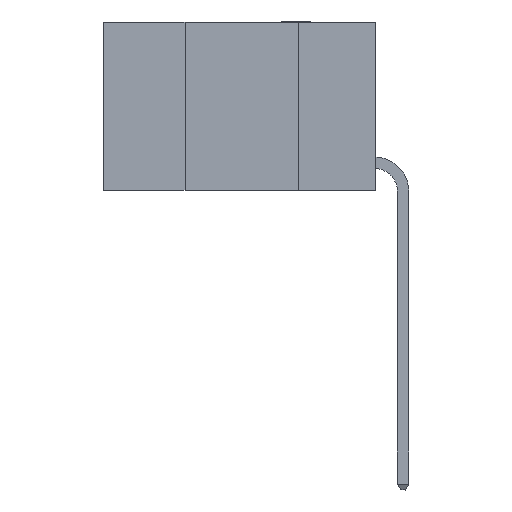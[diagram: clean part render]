
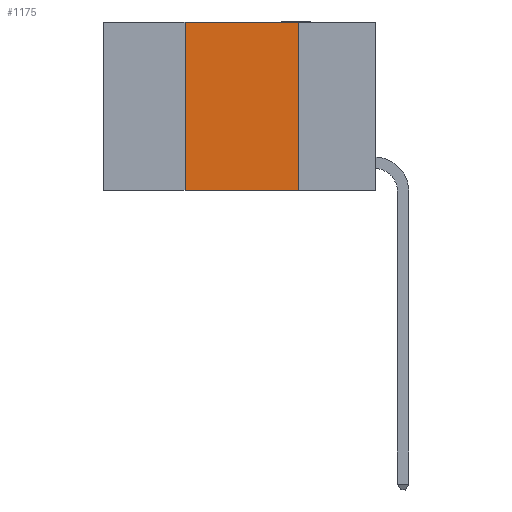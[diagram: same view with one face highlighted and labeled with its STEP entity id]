
A CAD part, left-side view. The second image highlights one B-rep face of the part: STEP entity #1175.
In plain terms, the highlighted planar face has unit normal (-1, 0, 0).
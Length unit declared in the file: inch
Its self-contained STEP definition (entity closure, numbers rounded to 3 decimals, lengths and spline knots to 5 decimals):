
#90 = FACE_OUTER_BOUND ( 'NONE', #10176, .T. ) ;
#216 = VERTEX_POINT ( 'NONE', #8531 ) ;
#694 = CARTESIAN_POINT ( 'NONE',  ( 0., 0.6, 0. ) ) ;
#1175 = ADVANCED_FACE ( 'NONE', ( #90 ), #14462, .F. ) ;
#1737 = VECTOR ( 'NONE', #1869, 39.37008 ) ;
#1763 = LINE ( 'NONE', #4527, #13417 ) ;
#1869 = DIRECTION ( 'NONE',  ( 0., -1., 0. ) ) ;
#3248 = EDGE_CURVE ( 'NONE', #9612, #3502, #7787, .T. ) ;
#3502 = VERTEX_POINT ( 'NONE', #4866 ) ;
#4141 = DIRECTION ( 'NONE',  ( 0., -1., 0. ) ) ;
#4346 = VECTOR ( 'NONE', #9895, 39.37008 ) ;
#4527 = CARTESIAN_POINT ( 'NONE',  ( 0., 0.17, 0. ) ) ;
#4866 = CARTESIAN_POINT ( 'NONE',  ( 0., 0.42, 0. ) ) ;
#6648 = ORIENTED_EDGE ( 'NONE', *, *, #3248, .F. ) ;
#7002 = EDGE_CURVE ( 'NONE', #3502, #216, #7847, .T. ) ;
#7080 = ORIENTED_EDGE ( 'NONE', *, *, #12931, .T. ) ;
#7787 = LINE ( 'NONE', #9945, #4346 ) ;
#7847 = LINE ( 'NONE', #694, #1737 ) ;
#7887 = EDGE_CURVE ( 'NONE', #216, #13329, #1763, .T. ) ;
#8531 = CARTESIAN_POINT ( 'NONE',  ( 0., 0.17, 0. ) ) ;
#8614 = LINE ( 'NONE', #12032, #14479 ) ;
#9342 = DIRECTION ( 'NONE',  ( 0., 0., -1. ) ) ;
#9573 = CARTESIAN_POINT ( 'NONE',  ( 0., 0.42, -0.37 ) ) ;
#9612 = VERTEX_POINT ( 'NONE', #9573 ) ;
#9776 = DIRECTION ( 'NONE',  ( 1., 0., 0. ) ) ;
#9895 = DIRECTION ( 'NONE',  ( 0., 0., 1. ) ) ;
#9945 = CARTESIAN_POINT ( 'NONE',  ( 0., 0.42, 0. ) ) ;
#10176 = EDGE_LOOP ( 'NONE', ( #10765, #11463, #6648, #7080 ) ) ;
#10345 = CARTESIAN_POINT ( 'NONE',  ( 0., 0.6, 0. ) ) ;
#10765 = ORIENTED_EDGE ( 'NONE', *, *, #7887, .F. ) ;
#11463 = ORIENTED_EDGE ( 'NONE', *, *, #7002, .F. ) ;
#11574 = CARTESIAN_POINT ( 'NONE',  ( 0., 0.17, -0.37 ) ) ;
#12032 = CARTESIAN_POINT ( 'NONE',  ( 0., 0.6, -0.37 ) ) ;
#12931 = EDGE_CURVE ( 'NONE', #9612, #13329, #8614, .T. ) ;
#13329 = VERTEX_POINT ( 'NONE', #11574 ) ;
#13417 = VECTOR ( 'NONE', #13534, 39.37008 ) ;
#13534 = DIRECTION ( 'NONE',  ( 0., 0., -1. ) ) ;
#14307 = AXIS2_PLACEMENT_3D ( 'NONE', #10345, #9776, #9342 ) ;
#14462 = PLANE ( 'NONE',  #14307 ) ;
#14479 = VECTOR ( 'NONE', #4141, 39.37008 ) ;
